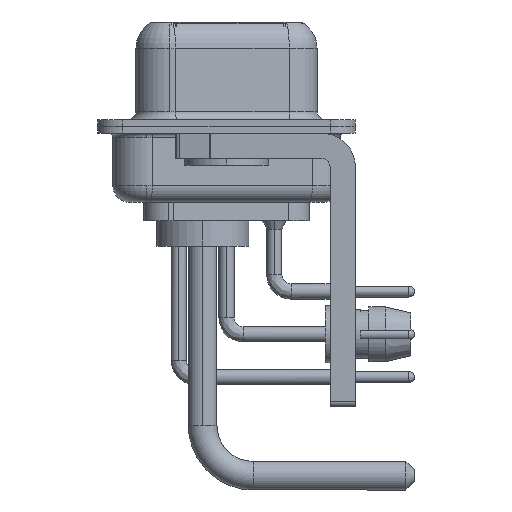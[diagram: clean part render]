
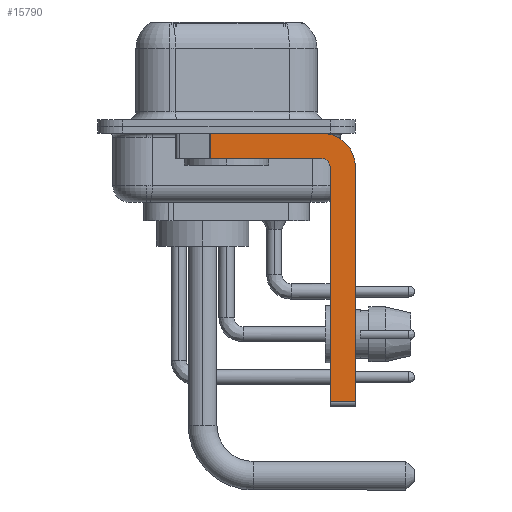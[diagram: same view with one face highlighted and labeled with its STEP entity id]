
A CAD part, left-side view. The second image highlights one B-rep face of the part: STEP entity #15790.
In plain terms, the highlighted planar face has unit normal (-1, 0, 0).
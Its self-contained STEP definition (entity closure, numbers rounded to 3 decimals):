
#97 = VECTOR ( 'NONE', #10362, 1000. ) ;
#162 = CARTESIAN_POINT ( 'NONE',  ( -2.9, -6.15, -2.4 ) ) ;
#842 = LINE ( 'NONE', #12074, #7531 ) ;
#1219 = AXIS2_PLACEMENT_3D ( 'NONE', #21160, #10269, #10449 ) ;
#1720 = ORIENTED_EDGE ( 'NONE', *, *, #18404, .F. ) ;
#1985 = ORIENTED_EDGE ( 'NONE', *, *, #18229, .F. ) ;
#2199 = CARTESIAN_POINT ( 'NONE',  ( -2.9, -5.65, -0.4 ) ) ;
#2429 = VECTOR ( 'NONE', #28822, 1000. ) ;
#2689 = DIRECTION ( 'NONE',  ( -1., 0., 0. ) ) ;
#3328 = DIRECTION ( 'NONE',  ( 0., -1., 0. ) ) ;
#5372 = LINE ( 'NONE', #27838, #8693 ) ;
#7531 = VECTOR ( 'NONE', #18268, 1000. ) ;
#7579 = CARTESIAN_POINT ( 'NONE',  ( -2.9, -5.65, -2.4 ) ) ;
#7638 = ORIENTED_EDGE ( 'NONE', *, *, #34306, .T. ) ;
#8447 = DIRECTION ( 'NONE',  ( 0., 0., 1. ) ) ;
#8693 = VECTOR ( 'NONE', #36085, 1000. ) ;
#8827 = VERTEX_POINT ( 'NONE', #32974 ) ;
#8862 = CARTESIAN_POINT ( 'NONE',  ( -2.9, 3., -0.4 ) ) ;
#9119 = LINE ( 'NONE', #31932, #2429 ) ;
#10269 = DIRECTION ( 'NONE',  ( 1., 0., 0. ) ) ;
#10362 = DIRECTION ( 'NONE',  ( 0., -1., 0. ) ) ;
#10449 = DIRECTION ( 'NONE',  ( 0., 0., -1. ) ) ;
#11214 = CARTESIAN_POINT ( 'NONE',  ( -2.9, -6.15, -16.6 ) ) ;
#12074 = CARTESIAN_POINT ( 'NONE',  ( -2.9, -5.65, -1.9 ) ) ;
#12132 = ORIENTED_EDGE ( 'NONE', *, *, #34228, .F. ) ;
#12487 = VERTEX_POINT ( 'NONE', #33302 ) ;
#13925 = DIRECTION ( 'NONE',  ( 0., 0., 1. ) ) ;
#14141 = VECTOR ( 'NONE', #3328, 1000. ) ;
#14146 = LINE ( 'NONE', #11214, #32847 ) ;
#15457 = VERTEX_POINT ( 'NONE', #35456 ) ;
#15790 = ADVANCED_FACE ( 'NONE', ( #30037 ), #27289, .F. ) ;
#16069 = CARTESIAN_POINT ( 'NONE',  ( -2.9, -7.65, -16.35 ) ) ;
#16490 = CIRCLE ( 'NONE', #25931, 0.5 ) ;
#16696 = ORIENTED_EDGE ( 'NONE', *, *, #19331, .F. ) ;
#17336 = LINE ( 'NONE', #8862, #14141 ) ;
#17847 = ORIENTED_EDGE ( 'NONE', *, *, #18989, .T. ) ;
#18103 = VERTEX_POINT ( 'NONE', #23551 ) ;
#18229 = EDGE_CURVE ( 'NONE', #20491, #8827, #31184, .T. ) ;
#18268 = DIRECTION ( 'NONE',  ( 0., 1., 0. ) ) ;
#18294 = LINE ( 'NONE', #24377, #97 ) ;
#18404 = EDGE_CURVE ( 'NONE', #33688, #12487, #16490, .T. ) ;
#18874 = ORIENTED_EDGE ( 'NONE', *, *, #34904, .F. ) ;
#18989 = EDGE_CURVE ( 'NONE', #18103, #36178, #18294, .T. ) ;
#19331 = EDGE_CURVE ( 'NONE', #21025, #20491, #17336, .T. ) ;
#20491 = VERTEX_POINT ( 'NONE', #2199 ) ;
#21025 = VERTEX_POINT ( 'NONE', #27929 ) ;
#21160 = CARTESIAN_POINT ( 'NONE',  ( -2.9, -5.65, -2.4 ) ) ;
#22145 = DIRECTION ( 'NONE',  ( 0., 0., -1. ) ) ;
#23551 = CARTESIAN_POINT ( 'NONE',  ( -2.9, -6.15, -16.35 ) ) ;
#24377 = CARTESIAN_POINT ( 'NONE',  ( -2.9, -5.65, -16.35 ) ) ;
#25931 = AXIS2_PLACEMENT_3D ( 'NONE', #30855, #2689, #13925 ) ;
#27289 = PLANE ( 'NONE',  #36304 ) ;
#27838 = CARTESIAN_POINT ( 'NONE',  ( -2.9, 0.978, -1.9 ) ) ;
#27929 = CARTESIAN_POINT ( 'NONE',  ( -2.9, 0.978, -0.4 ) ) ;
#27965 = EDGE_CURVE ( 'NONE', #8827, #36178, #9119, .T. ) ;
#28822 = DIRECTION ( 'NONE',  ( 0., 0., -1. ) ) ;
#30037 = FACE_OUTER_BOUND ( 'NONE', #34764, .T. ) ;
#30393 = DIRECTION ( 'NONE',  ( 1., 0., 0. ) ) ;
#30855 = CARTESIAN_POINT ( 'NONE',  ( -2.9, -5.65, -2.4 ) ) ;
#31184 = CIRCLE ( 'NONE', #1219, 2. ) ;
#31208 = ORIENTED_EDGE ( 'NONE', *, *, #27965, .F. ) ;
#31932 = CARTESIAN_POINT ( 'NONE',  ( -2.9, -7.65, -2.4 ) ) ;
#32847 = VECTOR ( 'NONE', #8447, 1000. ) ;
#32974 = CARTESIAN_POINT ( 'NONE',  ( -2.9, -7.65, -2.4 ) ) ;
#33302 = CARTESIAN_POINT ( 'NONE',  ( -2.9, -5.65, -1.9 ) ) ;
#33688 = VERTEX_POINT ( 'NONE', #162 ) ;
#34228 = EDGE_CURVE ( 'NONE', #12487, #15457, #842, .T. ) ;
#34306 = EDGE_CURVE ( 'NONE', #21025, #15457, #5372, .T. ) ;
#34764 = EDGE_LOOP ( 'NONE', ( #16696, #7638, #12132, #1720, #18874, #17847, #31208, #1985 ) ) ;
#34904 = EDGE_CURVE ( 'NONE', #18103, #33688, #14146, .T. ) ;
#35456 = CARTESIAN_POINT ( 'NONE',  ( -2.9, 0.978, -1.9 ) ) ;
#36085 = DIRECTION ( 'NONE',  ( 0., 0., -1. ) ) ;
#36178 = VERTEX_POINT ( 'NONE', #16069 ) ;
#36304 = AXIS2_PLACEMENT_3D ( 'NONE', #7579, #30393, #22145 ) ;
